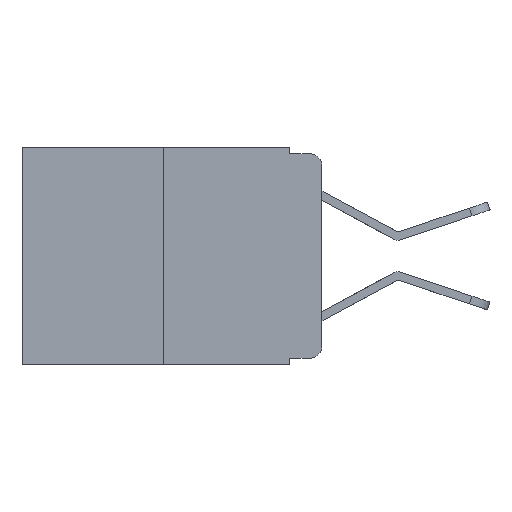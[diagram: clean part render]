
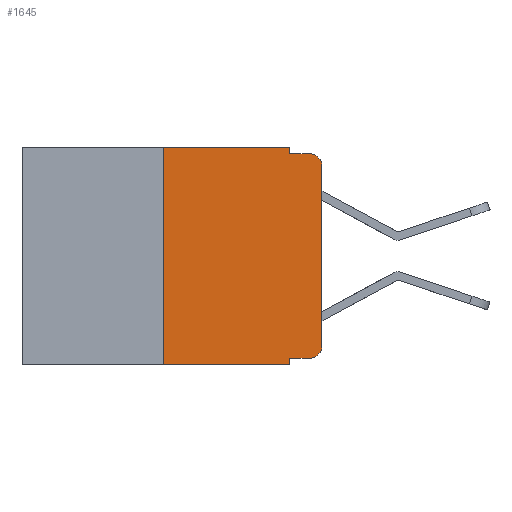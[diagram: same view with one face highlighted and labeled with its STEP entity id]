
A CAD part, left-side view. The second image highlights one B-rep face of the part: STEP entity #1645.
In plain terms, the highlighted planar face has unit normal (-1, 0, 0).
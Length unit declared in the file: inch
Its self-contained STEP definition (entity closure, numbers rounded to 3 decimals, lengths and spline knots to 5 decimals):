
#217 = EDGE_CURVE ( 'NONE', #14048, #12542, #8018, .T. ) ;
#298 = ORIENTED_EDGE ( 'NONE', *, *, #3791, .F. ) ;
#382 = CARTESIAN_POINT ( 'NONE',  ( 0., 0.02, -0.313 ) ) ;
#483 = EDGE_CURVE ( 'NONE', #16592, #10678, #2544, .T. ) ;
#588 = ORIENTED_EDGE ( 'NONE', *, *, #217, .F. ) ;
#799 = VECTOR ( 'NONE', #12518, 39.37008 ) ;
#818 = CARTESIAN_POINT ( 'NONE',  ( 0., 0.473, -0.343 ) ) ;
#1057 = LINE ( 'NONE', #6773, #13951 ) ;
#1192 = EDGE_CURVE ( 'NONE', #11597, #5095, #13138, .T. ) ;
#1202 = CARTESIAN_POINT ( 'NONE',  ( 0., 0.051, 0. ) ) ;
#1209 = VECTOR ( 'NONE', #11978, 39.37008 ) ;
#1468 = LINE ( 'NONE', #6830, #7814 ) ;
#1645 = ADVANCED_FACE ( 'NONE', ( #16763 ), #2816, .F. ) ;
#1683 = VECTOR ( 'NONE', #10935, 39.37008 ) ;
#2080 = CIRCLE ( 'NONE', #17273, 0.02 ) ;
#2544 = CIRCLE ( 'NONE', #14433, 0.02 ) ;
#2816 = PLANE ( 'NONE',  #17484 ) ;
#3010 = LINE ( 'NONE', #818, #799 ) ;
#3473 = DIRECTION ( 'NONE',  ( 0., -1., 0. ) ) ;
#3576 = CARTESIAN_POINT ( 'NONE',  ( 0., 0., 0. ) ) ;
#3610 = CARTESIAN_POINT ( 'NONE',  ( 0., 0.473, 0. ) ) ;
#3791 = EDGE_CURVE ( 'NONE', #9571, #5388, #1468, .T. ) ;
#4627 = EDGE_LOOP ( 'NONE', ( #14447, #16363, #7488, #298, #12371, #588, #11980, #6125, #11537, #17929 ) ) ;
#4663 = CARTESIAN_POINT ( 'NONE',  ( 0., 0.25, -0.343 ) ) ;
#4700 = CARTESIAN_POINT ( 'NONE',  ( 0., 0.051, -0.333 ) ) ;
#4713 = CARTESIAN_POINT ( 'NONE',  ( 0., 0., -0.03 ) ) ;
#4948 = DIRECTION ( 'NONE',  ( 0., -1., 0. ) ) ;
#4974 = CARTESIAN_POINT ( 'NONE',  ( 0., 0.051, -0.343 ) ) ;
#5095 = VERTEX_POINT ( 'NONE', #4974 ) ;
#5317 = EDGE_CURVE ( 'NONE', #11229, #7339, #2080, .T. ) ;
#5323 = EDGE_CURVE ( 'NONE', #11597, #11229, #17016, .T. ) ;
#5388 = VERTEX_POINT ( 'NONE', #5898 ) ;
#5816 = CARTESIAN_POINT ( 'NONE',  ( 0., 0.051, -0.333 ) ) ;
#5898 = CARTESIAN_POINT ( 'NONE',  ( 0., 0.051, -0.01 ) ) ;
#6010 = CARTESIAN_POINT ( 'NONE',  ( 0., 0.25, 0. ) ) ;
#6125 = ORIENTED_EDGE ( 'NONE', *, *, #1192, .F. ) ;
#6299 = DIRECTION ( 'NONE',  ( -1., 0., 0. ) ) ;
#6329 = CARTESIAN_POINT ( 'NONE',  ( 0., 0.02, -0.03 ) ) ;
#6773 = CARTESIAN_POINT ( 'NONE',  ( 0., 0.051, -0.01 ) ) ;
#6830 = CARTESIAN_POINT ( 'NONE',  ( 0., 0.051, 0. ) ) ;
#6885 = DIRECTION ( 'NONE',  ( 0., -1., 0. ) ) ;
#6947 = CARTESIAN_POINT ( 'NONE',  ( 0., 0.02, -0.01 ) ) ;
#7339 = VERTEX_POINT ( 'NONE', #9660 ) ;
#7488 = ORIENTED_EDGE ( 'NONE', *, *, #8746, .F. ) ;
#7783 = DIRECTION ( 'NONE',  ( -1., 0., 0. ) ) ;
#7814 = VECTOR ( 'NONE', #15656, 39.37008 ) ;
#7983 = VECTOR ( 'NONE', #3473, 39.37008 ) ;
#8018 = LINE ( 'NONE', #6010, #1209 ) ;
#8559 = DIRECTION ( 'NONE',  ( 0., 0., -1. ) ) ;
#8738 = CARTESIAN_POINT ( 'NONE',  ( 0., 0.051, 0. ) ) ;
#8742 = DIRECTION ( 'NONE',  ( 1., 0., 0. ) ) ;
#8746 = EDGE_CURVE ( 'NONE', #5388, #10678, #1057, .T. ) ;
#8944 = LINE ( 'NONE', #3576, #1683 ) ;
#9571 = VERTEX_POINT ( 'NONE', #1202 ) ;
#9660 = CARTESIAN_POINT ( 'NONE',  ( 0., 0., -0.313 ) ) ;
#10505 = DIRECTION ( 'NONE',  ( 0., 0., -1. ) ) ;
#10678 = VERTEX_POINT ( 'NONE', #6947 ) ;
#10935 = DIRECTION ( 'NONE',  ( 0., 0., 1. ) ) ;
#11229 = VERTEX_POINT ( 'NONE', #15117 ) ;
#11537 = ORIENTED_EDGE ( 'NONE', *, *, #5323, .T. ) ;
#11597 = VERTEX_POINT ( 'NONE', #5816 ) ;
#11978 = DIRECTION ( 'NONE',  ( 0., 0., 1. ) ) ;
#11980 = ORIENTED_EDGE ( 'NONE', *, *, #17893, .T. ) ;
#12070 = DIRECTION ( 'NONE',  ( 0., 0., -1. ) ) ;
#12346 = VECTOR ( 'NONE', #4948, 39.37008 ) ;
#12371 = ORIENTED_EDGE ( 'NONE', *, *, #13704, .F. ) ;
#12518 = DIRECTION ( 'NONE',  ( 0., -1., 0. ) ) ;
#12542 = VERTEX_POINT ( 'NONE', #15244 ) ;
#13138 = LINE ( 'NONE', #8738, #15873 ) ;
#13704 = EDGE_CURVE ( 'NONE', #12542, #9571, #15752, .T. ) ;
#13951 = VECTOR ( 'NONE', #6885, 39.37008 ) ;
#14048 = VERTEX_POINT ( 'NONE', #4663 ) ;
#14232 = EDGE_CURVE ( 'NONE', #7339, #16592, #8944, .T. ) ;
#14433 = AXIS2_PLACEMENT_3D ( 'NONE', #6329, #7783, #12070 ) ;
#14447 = ORIENTED_EDGE ( 'NONE', *, *, #14232, .T. ) ;
#15117 = CARTESIAN_POINT ( 'NONE',  ( 0., 0.02, -0.333 ) ) ;
#15244 = CARTESIAN_POINT ( 'NONE',  ( 0., 0.25, 0. ) ) ;
#15656 = DIRECTION ( 'NONE',  ( 0., 0., -1. ) ) ;
#15752 = LINE ( 'NONE', #3610, #12346 ) ;
#15873 = VECTOR ( 'NONE', #17131, 39.37008 ) ;
#16363 = ORIENTED_EDGE ( 'NONE', *, *, #483, .T. ) ;
#16592 = VERTEX_POINT ( 'NONE', #4713 ) ;
#16763 = FACE_OUTER_BOUND ( 'NONE', #4627, .T. ) ;
#17016 = LINE ( 'NONE', #4700, #7983 ) ;
#17131 = DIRECTION ( 'NONE',  ( 0., 0., -1. ) ) ;
#17273 = AXIS2_PLACEMENT_3D ( 'NONE', #382, #6299, #10505 ) ;
#17484 = AXIS2_PLACEMENT_3D ( 'NONE', #18752, #8742, #8559 ) ;
#17893 = EDGE_CURVE ( 'NONE', #14048, #5095, #3010, .T. ) ;
#17929 = ORIENTED_EDGE ( 'NONE', *, *, #5317, .T. ) ;
#18752 = CARTESIAN_POINT ( 'NONE',  ( 0., 0.473, 0. ) ) ;
